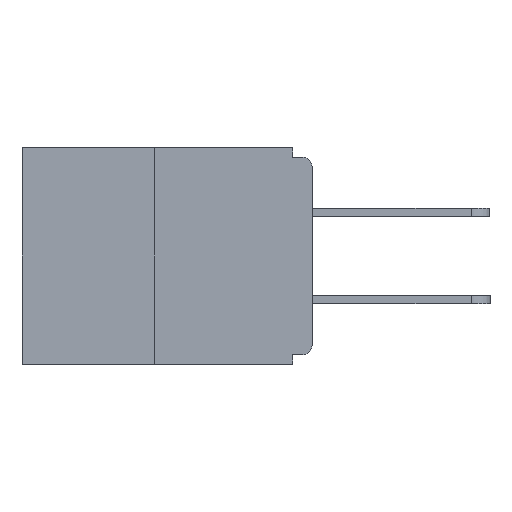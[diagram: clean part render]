
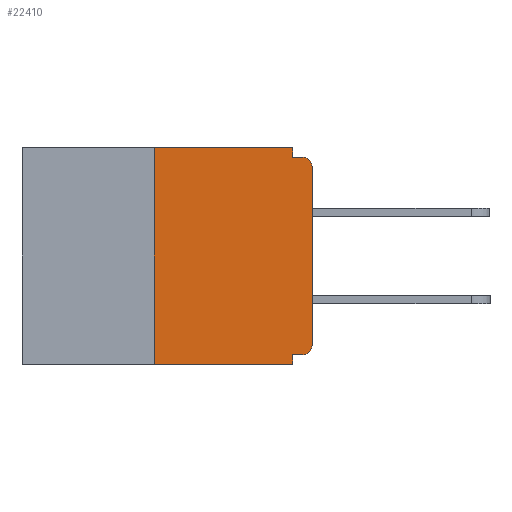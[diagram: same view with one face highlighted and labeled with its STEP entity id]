
A CAD part, left-side view. The second image highlights one B-rep face of the part: STEP entity #22410.
In plain terms, the highlighted planar face has unit normal (-1, 0, 0).
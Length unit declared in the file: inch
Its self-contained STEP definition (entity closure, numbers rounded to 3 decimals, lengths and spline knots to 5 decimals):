
#1048 = VERTEX_POINT ( 'NONE', #6970 ) ;
#1875 = VERTEX_POINT ( 'NONE', #31241 ) ;
#2039 = VECTOR ( 'NONE', #8566, 39.37008 ) ;
#2330 = LINE ( 'NONE', #31180, #18313 ) ;
#2785 = VERTEX_POINT ( 'NONE', #11064 ) ;
#3150 = VERTEX_POINT ( 'NONE', #8154 ) ;
#3333 = ORIENTED_EDGE ( 'NONE', *, *, #11893, .T. ) ;
#4393 = CIRCLE ( 'NONE', #20073, 0.015 ) ;
#4804 = CARTESIAN_POINT ( 'NONE',  ( 0., 0.031, -0.328 ) ) ;
#5131 = DIRECTION ( 'NONE',  ( 0., 0., 1. ) ) ;
#5478 = ORIENTED_EDGE ( 'NONE', *, *, #26435, .F. ) ;
#6432 = VECTOR ( 'NONE', #14043, 39.37008 ) ;
#6970 = CARTESIAN_POINT ( 'NONE',  ( 0., 0.031, -0.343 ) ) ;
#7061 = EDGE_CURVE ( 'NONE', #28419, #1875, #19380, .T. ) ;
#7768 = PLANE ( 'NONE',  #31273 ) ;
#8154 = CARTESIAN_POINT ( 'NONE',  ( 0., 0.015, -0.328 ) ) ;
#8417 = CARTESIAN_POINT ( 'NONE',  ( 0., 0.015, -0.03 ) ) ;
#8566 = DIRECTION ( 'NONE',  ( 0., -1., 0. ) ) ;
#8664 = CARTESIAN_POINT ( 'NONE',  ( 0., 0.46, -0.343 ) ) ;
#8810 = EDGE_CURVE ( 'NONE', #27532, #17544, #9034, .T. ) ;
#9034 = LINE ( 'NONE', #24462, #23850 ) ;
#9888 = EDGE_CURVE ( 'NONE', #17544, #26226, #25746, .T. ) ;
#10034 = LINE ( 'NONE', #8664, #2039 ) ;
#10549 = DIRECTION ( 'NONE',  ( 0., 0., -1. ) ) ;
#11014 = CARTESIAN_POINT ( 'NONE',  ( 0., 0.015, -0.313 ) ) ;
#11064 = CARTESIAN_POINT ( 'NONE',  ( 0., 0., -0.03 ) ) ;
#11372 = LINE ( 'NONE', #14368, #6432 ) ;
#11494 = CARTESIAN_POINT ( 'NONE',  ( 0., 0., 0. ) ) ;
#11875 = DIRECTION ( 'NONE',  ( 0., -1., 0. ) ) ;
#11893 = EDGE_CURVE ( 'NONE', #27532, #1048, #10034, .T. ) ;
#13935 = DIRECTION ( 'NONE',  ( 0., 0., 1. ) ) ;
#14043 = DIRECTION ( 'NONE',  ( 0., 0., -1. ) ) ;
#14205 = EDGE_CURVE ( 'NONE', #16338, #1048, #11372, .T. ) ;
#14368 = CARTESIAN_POINT ( 'NONE',  ( 0., 0.031, -0.343 ) ) ;
#15189 = FACE_OUTER_BOUND ( 'NONE', #21177, .T. ) ;
#15296 = ORIENTED_EDGE ( 'NONE', *, *, #22599, .T. ) ;
#15909 = VECTOR ( 'NONE', #20299, 39.37008 ) ;
#16338 = VERTEX_POINT ( 'NONE', #4804 ) ;
#17544 = VERTEX_POINT ( 'NONE', #25296 ) ;
#17580 = DIRECTION ( 'NONE',  ( 1., 0., 0. ) ) ;
#18313 = VECTOR ( 'NONE', #26186, 39.37008 ) ;
#18619 = CARTESIAN_POINT ( 'NONE',  ( 0., 0., -0.015 ) ) ;
#19046 = CARTESIAN_POINT ( 'NONE',  ( 0., 0.031, 0. ) ) ;
#19360 = VECTOR ( 'NONE', #13935, 39.37008 ) ;
#19380 = LINE ( 'NONE', #18619, #27404 ) ;
#19741 = CARTESIAN_POINT ( 'NONE',  ( 0., 0.46, 0. ) ) ;
#19790 = ORIENTED_EDGE ( 'NONE', *, *, #9888, .F. ) ;
#20073 = AXIS2_PLACEMENT_3D ( 'NONE', #11014, #20826, #25318 ) ;
#20223 = VERTEX_POINT ( 'NONE', #22695 ) ;
#20299 = DIRECTION ( 'NONE',  ( 0., 0., -1. ) ) ;
#20826 = DIRECTION ( 'NONE',  ( -1., 0., 0. ) ) ;
#21177 = EDGE_LOOP ( 'NONE', ( #19790, #26198, #3333, #27805, #25519, #28606, #28553, #15296, #23038, #5478 ) ) ;
#21475 = EDGE_CURVE ( 'NONE', #20223, #2785, #22437, .T. ) ;
#21870 = VECTOR ( 'NONE', #11875, 39.37008 ) ;
#22410 = ADVANCED_FACE ( 'NONE', ( #15189 ), #7768, .F. ) ;
#22437 = LINE ( 'NONE', #11494, #19360 ) ;
#22599 = EDGE_CURVE ( 'NONE', #2785, #1875, #25031, .T. ) ;
#22695 = CARTESIAN_POINT ( 'NONE',  ( 0., 0., -0.313 ) ) ;
#23038 = ORIENTED_EDGE ( 'NONE', *, *, #7061, .F. ) ;
#23382 = DIRECTION ( 'NONE',  ( 0., -1., 0. ) ) ;
#23457 = LINE ( 'NONE', #29790, #15909 ) ;
#23850 = VECTOR ( 'NONE', #5131, 39.37008 ) ;
#24115 = EDGE_CURVE ( 'NONE', #3150, #20223, #4393, .T. ) ;
#24462 = CARTESIAN_POINT ( 'NONE',  ( 0., 0.25, 0. ) ) ;
#24504 = CARTESIAN_POINT ( 'NONE',  ( 0., 0.25, -0.343 ) ) ;
#25031 = CIRCLE ( 'NONE', #29647, 0.015 ) ;
#25296 = CARTESIAN_POINT ( 'NONE',  ( 0., 0.25, 0. ) ) ;
#25318 = DIRECTION ( 'NONE',  ( 0., 0., -1. ) ) ;
#25519 = ORIENTED_EDGE ( 'NONE', *, *, #29583, .F. ) ;
#25746 = LINE ( 'NONE', #26301, #21870 ) ;
#26186 = DIRECTION ( 'NONE',  ( 0., 1., 0. ) ) ;
#26198 = ORIENTED_EDGE ( 'NONE', *, *, #8810, .F. ) ;
#26226 = VERTEX_POINT ( 'NONE', #19046 ) ;
#26301 = CARTESIAN_POINT ( 'NONE',  ( 0., 0.46, 0. ) ) ;
#26435 = EDGE_CURVE ( 'NONE', #26226, #28419, #23457, .T. ) ;
#27206 = DIRECTION ( 'NONE',  ( 0., 0., -1. ) ) ;
#27404 = VECTOR ( 'NONE', #23382, 39.37008 ) ;
#27532 = VERTEX_POINT ( 'NONE', #24504 ) ;
#27805 = ORIENTED_EDGE ( 'NONE', *, *, #14205, .F. ) ;
#27851 = DIRECTION ( 'NONE',  ( -1., 0., 0. ) ) ;
#28419 = VERTEX_POINT ( 'NONE', #30209 ) ;
#28553 = ORIENTED_EDGE ( 'NONE', *, *, #21475, .T. ) ;
#28606 = ORIENTED_EDGE ( 'NONE', *, *, #24115, .T. ) ;
#29583 = EDGE_CURVE ( 'NONE', #3150, #16338, #2330, .T. ) ;
#29647 = AXIS2_PLACEMENT_3D ( 'NONE', #8417, #27851, #10549 ) ;
#29790 = CARTESIAN_POINT ( 'NONE',  ( 0., 0.031, 0. ) ) ;
#30209 = CARTESIAN_POINT ( 'NONE',  ( 0., 0.031, -0.015 ) ) ;
#31180 = CARTESIAN_POINT ( 'NONE',  ( 0., 0., -0.328 ) ) ;
#31241 = CARTESIAN_POINT ( 'NONE',  ( 0., 0.015, -0.015 ) ) ;
#31273 = AXIS2_PLACEMENT_3D ( 'NONE', #19741, #17580, #27206 ) ;
